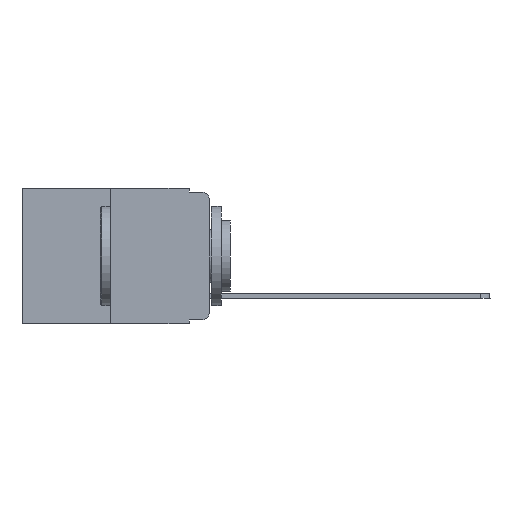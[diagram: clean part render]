
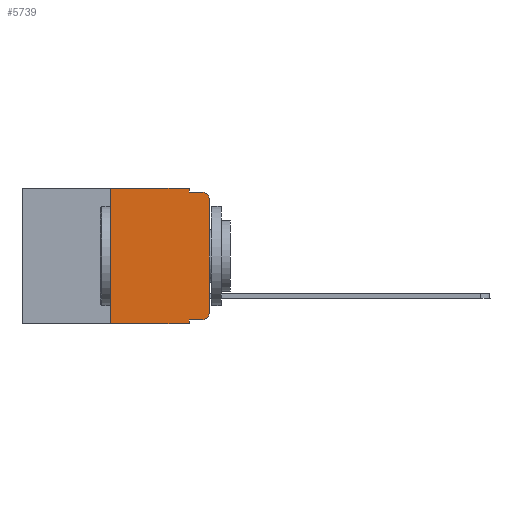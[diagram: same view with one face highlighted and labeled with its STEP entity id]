
A CAD part, left-side view. The second image highlights one B-rep face of the part: STEP entity #5739.
In plain terms, the highlighted planar face has unit normal (-1, 0, 0).
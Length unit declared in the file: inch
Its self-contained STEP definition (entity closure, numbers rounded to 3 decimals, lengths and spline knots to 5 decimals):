
#223 = CARTESIAN_POINT ( 'NONE',  ( 0., 0., 0. ) ) ;
#712 = PLANE ( 'NONE',  #16846 ) ;
#943 = DIRECTION ( 'NONE',  ( 0., -1., 0. ) ) ;
#1619 = CARTESIAN_POINT ( 'NONE',  ( 0., 0.051, -0.01 ) ) ;
#1777 = CIRCLE ( 'NONE', #7318, 0.02 ) ;
#1894 = VERTEX_POINT ( 'NONE', #18650 ) ;
#2046 = EDGE_CURVE ( 'NONE', #1894, #12148, #3201, .T. ) ;
#2331 = DIRECTION ( 'NONE',  ( 0., 0., -1. ) ) ;
#2796 = VERTEX_POINT ( 'NONE', #7307 ) ;
#2803 = EDGE_CURVE ( 'NONE', #3178, #12148, #11782, .T. ) ;
#3178 = VERTEX_POINT ( 'NONE', #10042 ) ;
#3201 = LINE ( 'NONE', #19849, #12573 ) ;
#3242 = ORIENTED_EDGE ( 'NONE', *, *, #2803, .T. ) ;
#3394 = VECTOR ( 'NONE', #5218, 39.37008 ) ;
#3638 = CIRCLE ( 'NONE', #18608, 0.02 ) ;
#3841 = DIRECTION ( 'NONE',  ( 0., -1., 0. ) ) ;
#3942 = CARTESIAN_POINT ( 'NONE',  ( 0., 0.473, 0. ) ) ;
#4276 = CARTESIAN_POINT ( 'NONE',  ( 0., 0.051, 0. ) ) ;
#4633 = CARTESIAN_POINT ( 'NONE',  ( 0., 0.473, 0. ) ) ;
#4848 = DIRECTION ( 'NONE',  ( 0., 0., -1. ) ) ;
#4892 = VECTOR ( 'NONE', #9196, 39.37008 ) ;
#5218 = DIRECTION ( 'NONE',  ( 0., -1., 0. ) ) ;
#5739 = ADVANCED_FACE ( 'NONE', ( #15289 ), #712, .F. ) ;
#6274 = CARTESIAN_POINT ( 'NONE',  ( 0., 0., -0.313 ) ) ;
#6446 = DIRECTION ( 'NONE',  ( 0., 0., -1. ) ) ;
#6654 = VERTEX_POINT ( 'NONE', #6274 ) ;
#6792 = VECTOR ( 'NONE', #943, 39.37008 ) ;
#6900 = VERTEX_POINT ( 'NONE', #15526 ) ;
#7088 = EDGE_CURVE ( 'NONE', #21308, #2796, #15160, .T. ) ;
#7090 = VERTEX_POINT ( 'NONE', #12383 ) ;
#7307 = CARTESIAN_POINT ( 'NONE',  ( 0., 0.02, -0.01 ) ) ;
#7318 = AXIS2_PLACEMENT_3D ( 'NONE', #19731, #14701, #6446 ) ;
#7564 = CARTESIAN_POINT ( 'NONE',  ( 0., 0.02, -0.333 ) ) ;
#8093 = LINE ( 'NONE', #4633, #17520 ) ;
#8230 = LINE ( 'NONE', #4276, #4892 ) ;
#8766 = VECTOR ( 'NONE', #17168, 39.37008 ) ;
#8794 = EDGE_LOOP ( 'NONE', ( #16299, #15528, #14780, #9823, #18180, #19022, #3242, #18008, #16062, #19901 ) ) ;
#9172 = CARTESIAN_POINT ( 'NONE',  ( 0., 0.02, -0.313 ) ) ;
#9196 = DIRECTION ( 'NONE',  ( 0., 0., -1. ) ) ;
#9272 = EDGE_CURVE ( 'NONE', #6654, #14994, #15307, .T. ) ;
#9823 = ORIENTED_EDGE ( 'NONE', *, *, #20124, .F. ) ;
#10042 = CARTESIAN_POINT ( 'NONE',  ( 0., 0.25, -0.343 ) ) ;
#10791 = DIRECTION ( 'NONE',  ( 0., 0., -1. ) ) ;
#11010 = CARTESIAN_POINT ( 'NONE',  ( 0., 0.25, 0. ) ) ;
#11782 = LINE ( 'NONE', #17175, #15717 ) ;
#12148 = VERTEX_POINT ( 'NONE', #17845 ) ;
#12230 = DIRECTION ( 'NONE',  ( 1., 0., 0. ) ) ;
#12383 = CARTESIAN_POINT ( 'NONE',  ( 0., 0.25, 0. ) ) ;
#12573 = VECTOR ( 'NONE', #4848, 39.37008 ) ;
#12608 = DIRECTION ( 'NONE',  ( 0., 0., 1. ) ) ;
#12753 = LINE ( 'NONE', #11010, #17197 ) ;
#13243 = VERTEX_POINT ( 'NONE', #7564 ) ;
#14650 = EDGE_CURVE ( 'NONE', #7090, #6900, #8093, .T. ) ;
#14701 = DIRECTION ( 'NONE',  ( -1., 0., 0. ) ) ;
#14780 = ORIENTED_EDGE ( 'NONE', *, *, #7088, .F. ) ;
#14994 = VERTEX_POINT ( 'NONE', #16156 ) ;
#15160 = LINE ( 'NONE', #20930, #6792 ) ;
#15289 = FACE_OUTER_BOUND ( 'NONE', #8794, .T. ) ;
#15307 = LINE ( 'NONE', #223, #8766 ) ;
#15526 = CARTESIAN_POINT ( 'NONE',  ( 0., 0.051, 0. ) ) ;
#15528 = ORIENTED_EDGE ( 'NONE', *, *, #19615, .T. ) ;
#15530 = EDGE_CURVE ( 'NONE', #1894, #13243, #16968, .T. ) ;
#15717 = VECTOR ( 'NONE', #3841, 39.37008 ) ;
#16062 = ORIENTED_EDGE ( 'NONE', *, *, #15530, .T. ) ;
#16156 = CARTESIAN_POINT ( 'NONE',  ( 0., 0., -0.03 ) ) ;
#16299 = ORIENTED_EDGE ( 'NONE', *, *, #9272, .T. ) ;
#16846 = AXIS2_PLACEMENT_3D ( 'NONE', #3942, #12230, #2331 ) ;
#16897 = CARTESIAN_POINT ( 'NONE',  ( 0., 0.051, -0.333 ) ) ;
#16968 = LINE ( 'NONE', #16897, #3394 ) ;
#17168 = DIRECTION ( 'NONE',  ( 0., 0., 1. ) ) ;
#17175 = CARTESIAN_POINT ( 'NONE',  ( 0., 0.473, -0.343 ) ) ;
#17197 = VECTOR ( 'NONE', #12608, 39.37008 ) ;
#17520 = VECTOR ( 'NONE', #19836, 39.37008 ) ;
#17845 = CARTESIAN_POINT ( 'NONE',  ( 0., 0.051, -0.343 ) ) ;
#18008 = ORIENTED_EDGE ( 'NONE', *, *, #2046, .F. ) ;
#18180 = ORIENTED_EDGE ( 'NONE', *, *, #14650, .F. ) ;
#18608 = AXIS2_PLACEMENT_3D ( 'NONE', #9172, #19014, #10791 ) ;
#18650 = CARTESIAN_POINT ( 'NONE',  ( 0., 0.051, -0.333 ) ) ;
#18765 = EDGE_CURVE ( 'NONE', #13243, #6654, #3638, .T. ) ;
#18828 = EDGE_CURVE ( 'NONE', #3178, #7090, #12753, .T. ) ;
#19014 = DIRECTION ( 'NONE',  ( -1., 0., 0. ) ) ;
#19022 = ORIENTED_EDGE ( 'NONE', *, *, #18828, .F. ) ;
#19615 = EDGE_CURVE ( 'NONE', #14994, #2796, #1777, .T. ) ;
#19731 = CARTESIAN_POINT ( 'NONE',  ( 0., 0.02, -0.03 ) ) ;
#19836 = DIRECTION ( 'NONE',  ( 0., -1., 0. ) ) ;
#19849 = CARTESIAN_POINT ( 'NONE',  ( 0., 0.051, 0. ) ) ;
#19901 = ORIENTED_EDGE ( 'NONE', *, *, #18765, .T. ) ;
#20124 = EDGE_CURVE ( 'NONE', #6900, #21308, #8230, .T. ) ;
#20930 = CARTESIAN_POINT ( 'NONE',  ( 0., 0.051, -0.01 ) ) ;
#21308 = VERTEX_POINT ( 'NONE', #1619 ) ;
